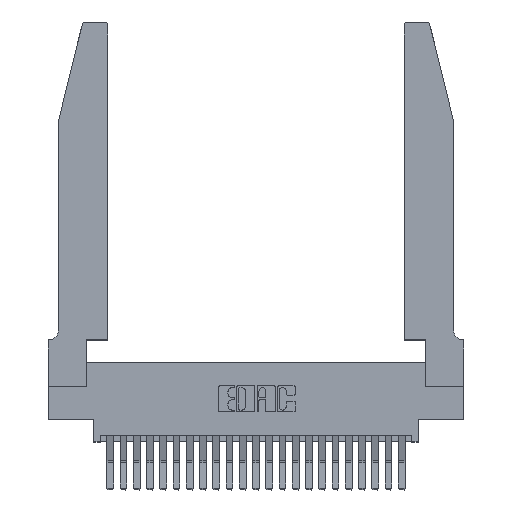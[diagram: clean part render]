
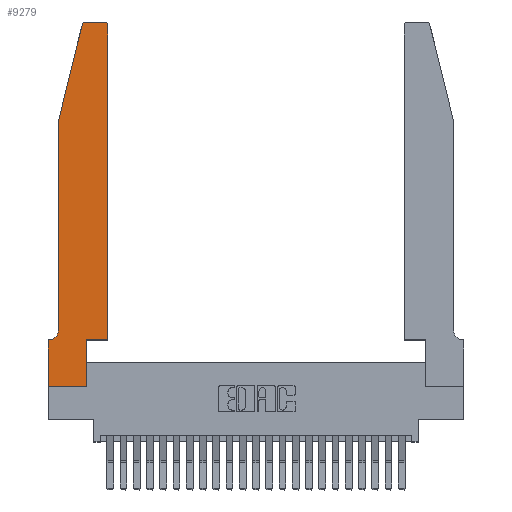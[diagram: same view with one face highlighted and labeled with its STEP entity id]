
A CAD part, top view. The second image highlights one B-rep face of the part: STEP entity #9279.
In plain terms, the highlighted planar face has unit normal (0, 0, 1).
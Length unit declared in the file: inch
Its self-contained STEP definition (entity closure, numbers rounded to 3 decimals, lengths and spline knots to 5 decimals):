
#39 = VECTOR ( 'NONE', #10389, 39.37008 ) ;
#654 = DIRECTION ( 'NONE',  ( 0., -1., 0. ) ) ;
#922 = LINE ( 'NONE', #19520, #4948 ) ;
#1114 = VERTEX_POINT ( 'NONE', #24967 ) ;
#1137 = VECTOR ( 'NONE', #10693, 39.37008 ) ;
#1146 = CARTESIAN_POINT ( 'NONE',  ( 0., 0.35, 0.37 ) ) ;
#1491 = FACE_OUTER_BOUND ( 'NONE', #8955, .T. ) ;
#1746 = LINE ( 'NONE', #6731, #1137 ) ;
#1769 = DIRECTION ( 'NONE',  ( 1., 0., 0. ) ) ;
#1819 = AXIS2_PLACEMENT_3D ( 'NONE', #18468, #6641, #20469 ) ;
#2284 = VERTEX_POINT ( 'NONE', #3874 ) ;
#2312 = CARTESIAN_POINT ( 'NONE',  ( 0., 0., 0.37 ) ) ;
#2424 = LINE ( 'NONE', #21754, #7706 ) ;
#2626 = ORIENTED_EDGE ( 'NONE', *, *, #25122, .T. ) ;
#3143 = DIRECTION ( 'NONE',  ( 1., 0., 0. ) ) ;
#3223 = DIRECTION ( 'NONE',  ( 0., 0., 1. ) ) ;
#3596 = CARTESIAN_POINT ( 'NONE',  ( 0.284, 2.75, 0.37 ) ) ;
#3641 = EDGE_CURVE ( 'NONE', #23382, #17435, #7304, .T. ) ;
#3815 = AXIS2_PLACEMENT_3D ( 'NONE', #25447, #13683, #1769 ) ;
#3874 = CARTESIAN_POINT ( 'NONE',  ( 0.25487, 2.72718, 0.37 ) ) ;
#3886 = DIRECTION ( 'NONE',  ( 1., 0., 0. ) ) ;
#4234 = VERTEX_POINT ( 'NONE', #25486 ) ;
#4948 = VECTOR ( 'NONE', #3886, 39.37008 ) ;
#5021 = LINE ( 'NONE', #10770, #25414 ) ;
#5400 = VERTEX_POINT ( 'NONE', #7488 ) ;
#6229 = CARTESIAN_POINT ( 'NONE',  ( 0.0055, 0.35, 0.37 ) ) ;
#6634 = CARTESIAN_POINT ( 'NONE',  ( 0., 0., 0.37 ) ) ;
#6641 = DIRECTION ( 'NONE',  ( 0., 0., -1. ) ) ;
#6677 = VECTOR ( 'NONE', #17170, 39.37008 ) ;
#6731 = CARTESIAN_POINT ( 'NONE',  ( 0.0755, 0.35, 0.37 ) ) ;
#6947 = EDGE_CURVE ( 'NONE', #17435, #4234, #5021, .T. ) ;
#6987 = CIRCLE ( 'NONE', #1819, 0.07 ) ;
#7304 = LINE ( 'NONE', #19139, #6677 ) ;
#7319 = CARTESIAN_POINT ( 'NONE',  ( 0., 0.35, 0.37 ) ) ;
#7488 = CARTESIAN_POINT ( 'NONE',  ( 0.0755, 0.42, 0.37 ) ) ;
#7593 = ORIENTED_EDGE ( 'NONE', *, *, #14639, .T. ) ;
#7706 = VECTOR ( 'NONE', #9944, 39.37008 ) ;
#8344 = EDGE_CURVE ( 'NONE', #23093, #1114, #922, .T. ) ;
#8417 = CARTESIAN_POINT ( 'NONE',  ( 0.2605, 2.75, 0.37 ) ) ;
#8955 = EDGE_LOOP ( 'NONE', ( #13036, #9916, #7593, #2626, #17126, #12365, #17578, #21377, #11977, #19865, #23386, #19152 ) ) ;
#8960 = VERTEX_POINT ( 'NONE', #3596 ) ;
#9279 = ADVANCED_FACE ( 'NONE', ( #1491 ), #13045, .T. ) ;
#9916 = ORIENTED_EDGE ( 'NONE', *, *, #17916, .T. ) ;
#9944 = DIRECTION ( 'NONE',  ( 0., 1., 0. ) ) ;
#10304 = VERTEX_POINT ( 'NONE', #6229 ) ;
#10389 = DIRECTION ( 'NONE',  ( -1., 0., 0. ) ) ;
#10693 = DIRECTION ( 'NONE',  ( -1., 0., 0. ) ) ;
#10770 = CARTESIAN_POINT ( 'NONE',  ( 0.4505, 0.35, 0.37 ) ) ;
#10801 = DIRECTION ( 'NONE',  ( -0.239, -0.971, 0. ) ) ;
#11457 = AXIS2_PLACEMENT_3D ( 'NONE', #15081, #3223, #17070 ) ;
#11832 = LINE ( 'NONE', #8417, #39 ) ;
#11857 = VECTOR ( 'NONE', #10801, 39.37008 ) ;
#11977 = ORIENTED_EDGE ( 'NONE', *, *, #16934, .T. ) ;
#12216 = VECTOR ( 'NONE', #24413, 39.37008 ) ;
#12365 = ORIENTED_EDGE ( 'NONE', *, *, #23256, .T. ) ;
#13036 = ORIENTED_EDGE ( 'NONE', *, *, #20494, .T. ) ;
#13045 = PLANE ( 'NONE',  #15296 ) ;
#13161 = CARTESIAN_POINT ( 'NONE',  ( 0.2865, 0.35, 0.37 ) ) ;
#13471 = LINE ( 'NONE', #24326, #22688 ) ;
#13683 = DIRECTION ( 'NONE',  ( 0., 0., 1. ) ) ;
#14469 = CIRCLE ( 'NONE', #3815, 0.03 ) ;
#14639 = EDGE_CURVE ( 'NONE', #2284, #15480, #17110, .T. ) ;
#15004 = DIRECTION ( 'NONE',  ( 0., 0., 1. ) ) ;
#15081 = CARTESIAN_POINT ( 'NONE',  ( 0.4205, 2.72, 0.37 ) ) ;
#15296 = AXIS2_PLACEMENT_3D ( 'NONE', #1146, #15004, #3143 ) ;
#15480 = VERTEX_POINT ( 'NONE', #18807 ) ;
#15558 = VERTEX_POINT ( 'NONE', #7319 ) ;
#16686 = CARTESIAN_POINT ( 'NONE',  ( 0.0755, 2., 0.37 ) ) ;
#16741 = DIRECTION ( 'NONE',  ( 0., 1., 0. ) ) ;
#16934 = EDGE_CURVE ( 'NONE', #1114, #23382, #2424, .T. ) ;
#17070 = DIRECTION ( 'NONE',  ( 1., 0., 0. ) ) ;
#17110 = LINE ( 'NONE', #16686, #11857 ) ;
#17126 = ORIENTED_EDGE ( 'NONE', *, *, #19417, .T. ) ;
#17170 = DIRECTION ( 'NONE',  ( 1., 0., 0. ) ) ;
#17435 = VERTEX_POINT ( 'NONE', #23126 ) ;
#17578 = ORIENTED_EDGE ( 'NONE', *, *, #25130, .T. ) ;
#17815 = CIRCLE ( 'NONE', #11457, 0.03 ) ;
#17916 = EDGE_CURVE ( 'NONE', #8960, #2284, #14469, .T. ) ;
#18069 = LINE ( 'NONE', #6634, #12216 ) ;
#18468 = CARTESIAN_POINT ( 'NONE',  ( 0.0055, 0.42, 0.37 ) ) ;
#18807 = CARTESIAN_POINT ( 'NONE',  ( 0.0755, 2., 0.37 ) ) ;
#19139 = CARTESIAN_POINT ( 'NONE',  ( 0.4505, 0.35, 0.37 ) ) ;
#19152 = ORIENTED_EDGE ( 'NONE', *, *, #23938, .T. ) ;
#19417 = EDGE_CURVE ( 'NONE', #5400, #10304, #6987, .T. ) ;
#19520 = CARTESIAN_POINT ( 'NONE',  ( 0., 0., 0.37 ) ) ;
#19865 = ORIENTED_EDGE ( 'NONE', *, *, #3641, .T. ) ;
#20469 = DIRECTION ( 'NONE',  ( -1., 0., 0. ) ) ;
#20494 = EDGE_CURVE ( 'NONE', #25562, #8960, #11832, .T. ) ;
#21377 = ORIENTED_EDGE ( 'NONE', *, *, #8344, .T. ) ;
#21754 = CARTESIAN_POINT ( 'NONE',  ( 0.2865, 0.35, 0.37 ) ) ;
#22235 = CARTESIAN_POINT ( 'NONE',  ( 0.4205, 2.75, 0.37 ) ) ;
#22688 = VECTOR ( 'NONE', #654, 39.37008 ) ;
#23093 = VERTEX_POINT ( 'NONE', #2312 ) ;
#23126 = CARTESIAN_POINT ( 'NONE',  ( 0.4505, 0.35, 0.37 ) ) ;
#23256 = EDGE_CURVE ( 'NONE', #10304, #15558, #1746, .T. ) ;
#23382 = VERTEX_POINT ( 'NONE', #13161 ) ;
#23386 = ORIENTED_EDGE ( 'NONE', *, *, #6947, .T. ) ;
#23938 = EDGE_CURVE ( 'NONE', #4234, #25562, #17815, .T. ) ;
#24326 = CARTESIAN_POINT ( 'NONE',  ( 0.0755, 2., 0.37 ) ) ;
#24413 = DIRECTION ( 'NONE',  ( 0., -1., 0. ) ) ;
#24967 = CARTESIAN_POINT ( 'NONE',  ( 0.2865, 0., 0.37 ) ) ;
#25122 = EDGE_CURVE ( 'NONE', #15480, #5400, #13471, .T. ) ;
#25130 = EDGE_CURVE ( 'NONE', #15558, #23093, #18069, .T. ) ;
#25414 = VECTOR ( 'NONE', #16741, 39.37008 ) ;
#25447 = CARTESIAN_POINT ( 'NONE',  ( 0.284, 2.72, 0.37 ) ) ;
#25486 = CARTESIAN_POINT ( 'NONE',  ( 0.4505, 2.72, 0.37 ) ) ;
#25562 = VERTEX_POINT ( 'NONE', #22235 ) ;
